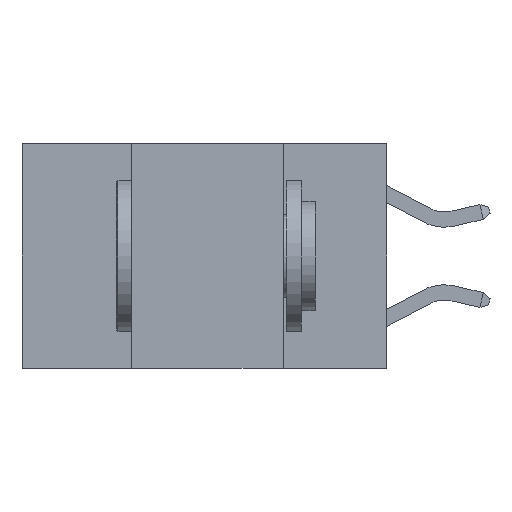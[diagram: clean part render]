
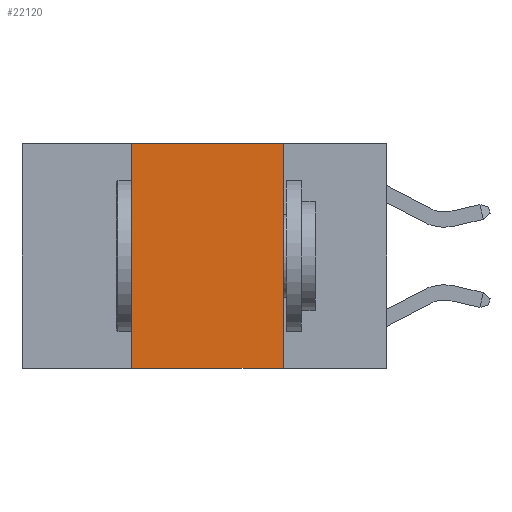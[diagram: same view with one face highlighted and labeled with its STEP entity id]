
A CAD part, left-side view. The second image highlights one B-rep face of the part: STEP entity #22120.
In plain terms, the highlighted planar face has unit normal (-1, 0, 0).
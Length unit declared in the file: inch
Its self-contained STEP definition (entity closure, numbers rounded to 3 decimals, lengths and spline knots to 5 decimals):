
#47 = DIRECTION ( 'NONE',  ( 0., -1., 0. ) ) ;
#189 = CARTESIAN_POINT ( 'NONE',  ( 0., 0.42, 0. ) ) ;
#993 = AXIS2_PLACEMENT_3D ( 'NONE', #9206, #22578, #13358 ) ;
#1588 = CARTESIAN_POINT ( 'NONE',  ( 0., 0.6, 0. ) ) ;
#1640 = LINE ( 'NONE', #28291, #15928 ) ;
#6142 = DIRECTION ( 'NONE',  ( 0., 0., -1. ) ) ;
#7210 = VECTOR ( 'NONE', #13398, 39.37008 ) ;
#8236 = EDGE_CURVE ( 'NONE', #10466, #24816, #8808, .T. ) ;
#8434 = ORIENTED_EDGE ( 'NONE', *, *, #8236, .T. ) ;
#8808 = LINE ( 'NONE', #22179, #14977 ) ;
#8834 = ORIENTED_EDGE ( 'NONE', *, *, #23797, .F. ) ;
#9206 = CARTESIAN_POINT ( 'NONE',  ( 0., 0.6, 0. ) ) ;
#9539 = CARTESIAN_POINT ( 'NONE',  ( 0., 0.17, -0.37 ) ) ;
#9676 = VERTEX_POINT ( 'NONE', #189 ) ;
#10252 = ORIENTED_EDGE ( 'NONE', *, *, #17608, .F. ) ;
#10466 = VERTEX_POINT ( 'NONE', #21824 ) ;
#10658 = DIRECTION ( 'NONE',  ( 0., -1., 0. ) ) ;
#13358 = DIRECTION ( 'NONE',  ( 0., 0., -1. ) ) ;
#13398 = DIRECTION ( 'NONE',  ( 0., 0., 1. ) ) ;
#14977 = VECTOR ( 'NONE', #47, 39.37008 ) ;
#15623 = LINE ( 'NONE', #29205, #7210 ) ;
#15727 = PLANE ( 'NONE',  #993 ) ;
#15928 = VECTOR ( 'NONE', #6142, 39.37008 ) ;
#16172 = FACE_OUTER_BOUND ( 'NONE', #21587, .T. ) ;
#17608 = EDGE_CURVE ( 'NONE', #25822, #24816, #1640, .T. ) ;
#21587 = EDGE_LOOP ( 'NONE', ( #10252, #8834, #27449, #8434 ) ) ;
#21824 = CARTESIAN_POINT ( 'NONE',  ( 0., 0.42, -0.37 ) ) ;
#21958 = LINE ( 'NONE', #1588, #23861 ) ;
#22120 = ADVANCED_FACE ( 'NONE', ( #16172 ), #15727, .F. ) ;
#22179 = CARTESIAN_POINT ( 'NONE',  ( 0., 0.6, -0.37 ) ) ;
#22578 = DIRECTION ( 'NONE',  ( 1., 0., 0. ) ) ;
#22865 = EDGE_CURVE ( 'NONE', #10466, #9676, #15623, .T. ) ;
#23797 = EDGE_CURVE ( 'NONE', #9676, #25822, #21958, .T. ) ;
#23861 = VECTOR ( 'NONE', #10658, 39.37008 ) ;
#24816 = VERTEX_POINT ( 'NONE', #9539 ) ;
#25822 = VERTEX_POINT ( 'NONE', #28355 ) ;
#27449 = ORIENTED_EDGE ( 'NONE', *, *, #22865, .F. ) ;
#28291 = CARTESIAN_POINT ( 'NONE',  ( 0., 0.17, 0. ) ) ;
#28355 = CARTESIAN_POINT ( 'NONE',  ( 0., 0.17, 0. ) ) ;
#29205 = CARTESIAN_POINT ( 'NONE',  ( 0., 0.42, 0. ) ) ;
